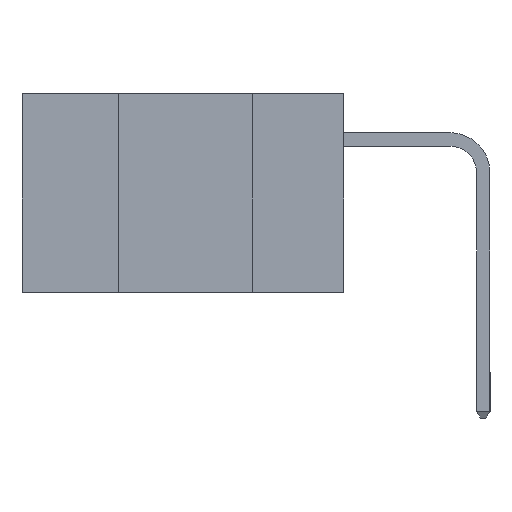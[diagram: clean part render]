
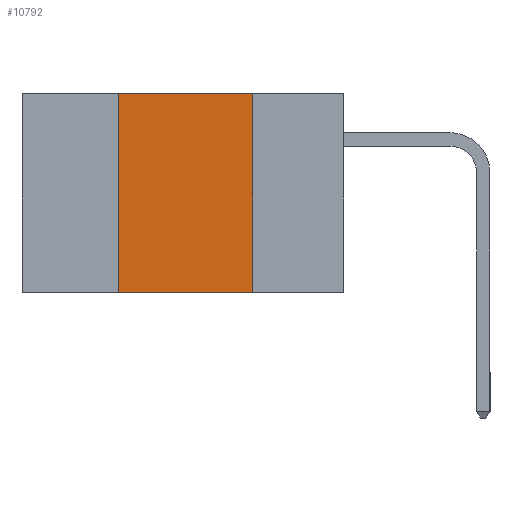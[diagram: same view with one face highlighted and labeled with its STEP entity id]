
A CAD part, left-side view. The second image highlights one B-rep face of the part: STEP entity #10792.
In plain terms, the highlighted planar face has unit normal (-1, 0, 0).
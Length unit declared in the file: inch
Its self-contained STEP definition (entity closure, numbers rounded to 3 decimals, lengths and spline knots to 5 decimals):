
#338 = VERTEX_POINT ( 'NONE', #16427 ) ;
#774 = LINE ( 'NONE', #11104, #11116 ) ;
#2913 = CARTESIAN_POINT ( 'NONE',  ( 0., 0.17, 0. ) ) ;
#3287 = AXIS2_PLACEMENT_3D ( 'NONE', #16052, #16289, #4518 ) ;
#3685 = LINE ( 'NONE', #7655, #12720 ) ;
#3687 = LINE ( 'NONE', #5063, #11306 ) ;
#4080 = CARTESIAN_POINT ( 'NONE',  ( 0., 0.17, -0.37 ) ) ;
#4518 = DIRECTION ( 'NONE',  ( 0., 0., -1. ) ) ;
#5063 = CARTESIAN_POINT ( 'NONE',  ( 0., 0.42, -0.37 ) ) ;
#6132 = ORIENTED_EDGE ( 'NONE', *, *, #13006, .F. ) ;
#6528 = CARTESIAN_POINT ( 'NONE',  ( 0., 0.6, -0.37 ) ) ;
#6784 = CARTESIAN_POINT ( 'NONE',  ( 0., 0.42, 0. ) ) ;
#7557 = DIRECTION ( 'NONE',  ( 0., -1., 0. ) ) ;
#7655 = CARTESIAN_POINT ( 'NONE',  ( 0., 0.6, 0. ) ) ;
#7836 = ORIENTED_EDGE ( 'NONE', *, *, #9958, .T. ) ;
#8446 = VERTEX_POINT ( 'NONE', #2913 ) ;
#8499 = DIRECTION ( 'NONE',  ( 0., 0., -1. ) ) ;
#8745 = EDGE_LOOP ( 'NONE', ( #12797, #16131, #6132, #7836 ) ) ;
#8927 = LINE ( 'NONE', #6528, #11858 ) ;
#9958 = EDGE_CURVE ( 'NONE', #338, #11004, #8927, .T. ) ;
#10322 = DIRECTION ( 'NONE',  ( 0., 0., 1. ) ) ;
#10647 = VERTEX_POINT ( 'NONE', #6784 ) ;
#10792 = ADVANCED_FACE ( 'NONE', ( #10816 ), #11069, .F. ) ;
#10816 = FACE_OUTER_BOUND ( 'NONE', #8745, .T. ) ;
#11004 = VERTEX_POINT ( 'NONE', #4080 ) ;
#11069 = PLANE ( 'NONE',  #3287 ) ;
#11104 = CARTESIAN_POINT ( 'NONE',  ( 0., 0.17, -0.37 ) ) ;
#11116 = VECTOR ( 'NONE', #8499, 39.37008 ) ;
#11306 = VECTOR ( 'NONE', #10322, 39.37008 ) ;
#11858 = VECTOR ( 'NONE', #7557, 39.37008 ) ;
#12720 = VECTOR ( 'NONE', #12893, 39.37008 ) ;
#12797 = ORIENTED_EDGE ( 'NONE', *, *, #15960, .F. ) ;
#12893 = DIRECTION ( 'NONE',  ( 0., -1., 0. ) ) ;
#13006 = EDGE_CURVE ( 'NONE', #338, #10647, #3687, .T. ) ;
#14779 = EDGE_CURVE ( 'NONE', #10647, #8446, #3685, .T. ) ;
#15960 = EDGE_CURVE ( 'NONE', #8446, #11004, #774, .T. ) ;
#16052 = CARTESIAN_POINT ( 'NONE',  ( 0., 0.6, 0. ) ) ;
#16131 = ORIENTED_EDGE ( 'NONE', *, *, #14779, .F. ) ;
#16289 = DIRECTION ( 'NONE',  ( 1., 0., 0. ) ) ;
#16427 = CARTESIAN_POINT ( 'NONE',  ( 0., 0.42, -0.37 ) ) ;
